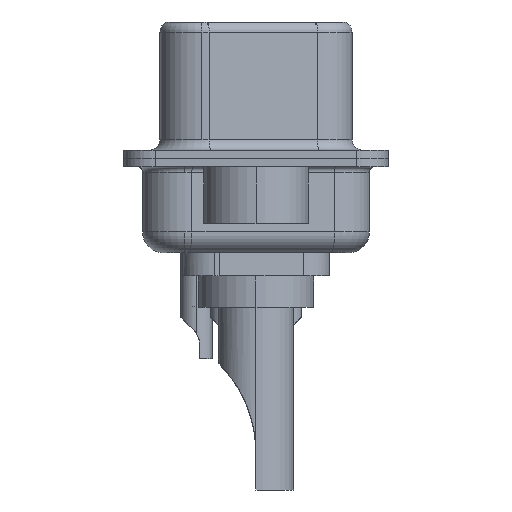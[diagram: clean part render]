
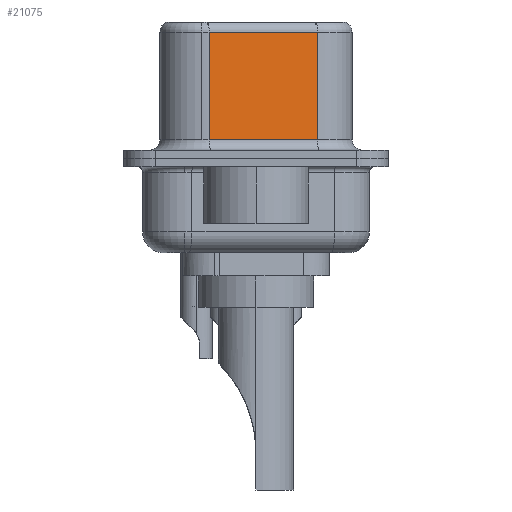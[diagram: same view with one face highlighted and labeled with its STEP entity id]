
A CAD part, left-side view. The second image highlights one B-rep face of the part: STEP entity #21075.
In plain terms, the highlighted planar face has unit normal (-0.985, -0.174, 0).
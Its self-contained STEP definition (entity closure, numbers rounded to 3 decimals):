
#495 = DIRECTION ( 'NONE',  ( 0., 0., -1. ) ) ;
#609 = CARTESIAN_POINT ( 'NONE',  ( 3.67, 2.233, 6.52 ) ) ;
#2205 = LINE ( 'NONE', #19712, #11880 ) ;
#2278 = EDGE_CURVE ( 'NONE', #4473, #10384, #7095, .T. ) ;
#2751 = EDGE_CURVE ( 'NONE', #4701, #4473, #2205, .T. ) ;
#2943 = ORIENTED_EDGE ( 'NONE', *, *, #17432, .T. ) ;
#2957 = AXIS2_PLACEMENT_3D ( 'NONE', #18779, #10118, #22271 ) ;
#3205 = EDGE_LOOP ( 'NONE', ( #9727, #11962, #21821, #2943 ) ) ;
#3591 = CARTESIAN_POINT ( 'NONE',  ( 3.67, 2.233, 6.02 ) ) ;
#4473 = VERTEX_POINT ( 'NONE', #3591 ) ;
#4701 = VERTEX_POINT ( 'NONE', #15340 ) ;
#7095 = LINE ( 'NONE', #609, #16420 ) ;
#8063 = DIRECTION ( 'NONE',  ( 0.174, -0.985, 0. ) ) ;
#8374 = VECTOR ( 'NONE', #20316, 1000. ) ;
#9727 = ORIENTED_EDGE ( 'NONE', *, *, #18877, .F. ) ;
#10118 = DIRECTION ( 'NONE',  ( 0.985, 0.174, 0. ) ) ;
#10244 = CARTESIAN_POINT ( 'NONE',  ( 4.58, -2.927, 0.9 ) ) ;
#10384 = VERTEX_POINT ( 'NONE', #22198 ) ;
#11880 = VECTOR ( 'NONE', #18346, 1000. ) ;
#11962 = ORIENTED_EDGE ( 'NONE', *, *, #2751, .T. ) ;
#12160 = VERTEX_POINT ( 'NONE', #10244 ) ;
#13340 = CARTESIAN_POINT ( 'NONE',  ( 4.58, -2.927, 0.9 ) ) ;
#13964 = VECTOR ( 'NONE', #8063, 1000. ) ;
#15340 = CARTESIAN_POINT ( 'NONE',  ( 4.58, -2.927, 6.02 ) ) ;
#16420 = VECTOR ( 'NONE', #495, 1000. ) ;
#16772 = FACE_OUTER_BOUND ( 'NONE', #3205, .T. ) ;
#17432 = EDGE_CURVE ( 'NONE', #10384, #12160, #18522, .T. ) ;
#18346 = DIRECTION ( 'NONE',  ( -0.174, 0.985, 0. ) ) ;
#18522 = LINE ( 'NONE', #13340, #13964 ) ;
#18709 = PLANE ( 'NONE',  #2957 ) ;
#18779 = CARTESIAN_POINT ( 'NONE',  ( 4.58, -2.927, 6.52 ) ) ;
#18877 = EDGE_CURVE ( 'NONE', #4701, #12160, #22278, .T. ) ;
#19712 = CARTESIAN_POINT ( 'NONE',  ( 4.58, -2.927, 6.02 ) ) ;
#20316 = DIRECTION ( 'NONE',  ( 0., 0., -1. ) ) ;
#21075 = ADVANCED_FACE ( 'NONE', ( #16772 ), #18709, .F. ) ;
#21821 = ORIENTED_EDGE ( 'NONE', *, *, #2278, .T. ) ;
#22041 = CARTESIAN_POINT ( 'NONE',  ( 4.58, -2.927, 6.52 ) ) ;
#22198 = CARTESIAN_POINT ( 'NONE',  ( 3.67, 2.233, 0.9 ) ) ;
#22271 = DIRECTION ( 'NONE',  ( -0.174, 0.985, 0. ) ) ;
#22278 = LINE ( 'NONE', #22041, #8374 ) ;
